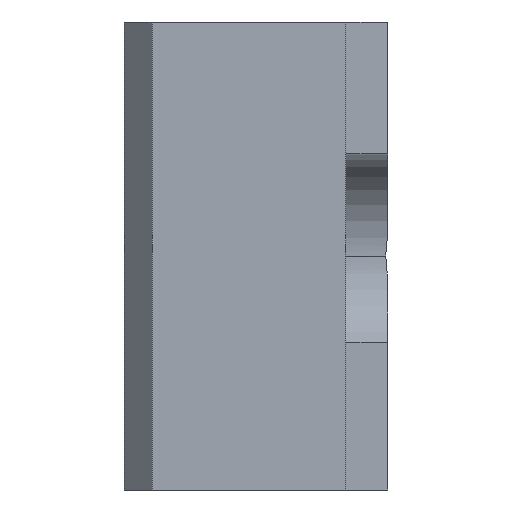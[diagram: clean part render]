
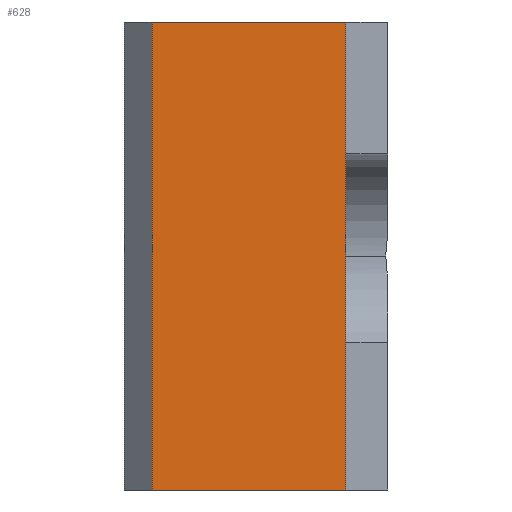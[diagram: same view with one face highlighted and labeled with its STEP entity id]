
A CAD part, front view. The second image highlights one B-rep face of the part: STEP entity #628.
In plain terms, the highlighted planar face has unit normal (0, -1, 0).
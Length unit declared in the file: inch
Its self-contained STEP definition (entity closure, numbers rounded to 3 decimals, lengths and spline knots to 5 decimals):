
#1 = AXIS2_PLACEMENT_3D ( 'NONE', #301, #355, #253 ) ;
#63 = VECTOR ( 'NONE', #572, 39.37008 ) ;
#72 = VECTOR ( 'NONE', #512, 39.37008 ) ;
#140 = ORIENTED_EDGE ( 'NONE', *, *, #576, .F. ) ;
#165 = CARTESIAN_POINT ( 'NONE',  ( -0.90714, -0.257, 0.6 ) ) ;
#168 = LINE ( 'NONE', #584, #774 ) ;
#204 = FACE_OUTER_BOUND ( 'NONE', #328, .T. ) ;
#213 = LINE ( 'NONE', #486, #285 ) ;
#232 = VERTEX_POINT ( 'NONE', #670 ) ;
#237 = DIRECTION ( 'NONE',  ( 1., 0., 0. ) ) ;
#240 = VERTEX_POINT ( 'NONE', #368 ) ;
#253 = DIRECTION ( 'NONE',  ( -1., 0., 0. ) ) ;
#285 = VECTOR ( 'NONE', #296, 39.37008 ) ;
#296 = DIRECTION ( 'NONE',  ( 0., 0., -1. ) ) ;
#301 = CARTESIAN_POINT ( 'NONE',  ( -0.90714, -0.257, 0.6 ) ) ;
#308 = VERTEX_POINT ( 'NONE', #322 ) ;
#322 = CARTESIAN_POINT ( 'NONE',  ( -0.6585, -0.257, 0. ) ) ;
#328 = EDGE_LOOP ( 'NONE', ( #446, #539, #140, #629 ) ) ;
#355 = DIRECTION ( 'NONE',  ( 0., 1., 0. ) ) ;
#368 = CARTESIAN_POINT ( 'NONE',  ( -0.90714, -0.257, 0. ) ) ;
#414 = EDGE_CURVE ( 'NONE', #654, #240, #753, .T. ) ;
#428 = LINE ( 'NONE', #748, #72 ) ;
#446 = ORIENTED_EDGE ( 'NONE', *, *, #461, .T. ) ;
#461 = EDGE_CURVE ( 'NONE', #240, #308, #428, .T. ) ;
#486 = CARTESIAN_POINT ( 'NONE',  ( -0.6585, -0.257, 0.6 ) ) ;
#512 = DIRECTION ( 'NONE',  ( 1., 0., 0. ) ) ;
#535 = PLANE ( 'NONE',  #1 ) ;
#537 = CARTESIAN_POINT ( 'NONE',  ( -0.90714, -0.257, 0.6 ) ) ;
#539 = ORIENTED_EDGE ( 'NONE', *, *, #749, .F. ) ;
#572 = DIRECTION ( 'NONE',  ( 0., 0., -1. ) ) ;
#576 = EDGE_CURVE ( 'NONE', #654, #232, #168, .T. ) ;
#584 = CARTESIAN_POINT ( 'NONE',  ( -0.90714, -0.257, 0.6 ) ) ;
#628 = ADVANCED_FACE ( 'NONE', ( #204 ), #535, .F. ) ;
#629 = ORIENTED_EDGE ( 'NONE', *, *, #414, .T. ) ;
#654 = VERTEX_POINT ( 'NONE', #537 ) ;
#670 = CARTESIAN_POINT ( 'NONE',  ( -0.6585, -0.257, 0.6 ) ) ;
#748 = CARTESIAN_POINT ( 'NONE',  ( -0.90714, -0.257, 0. ) ) ;
#749 = EDGE_CURVE ( 'NONE', #232, #308, #213, .T. ) ;
#753 = LINE ( 'NONE', #165, #63 ) ;
#774 = VECTOR ( 'NONE', #237, 39.37008 ) ;
